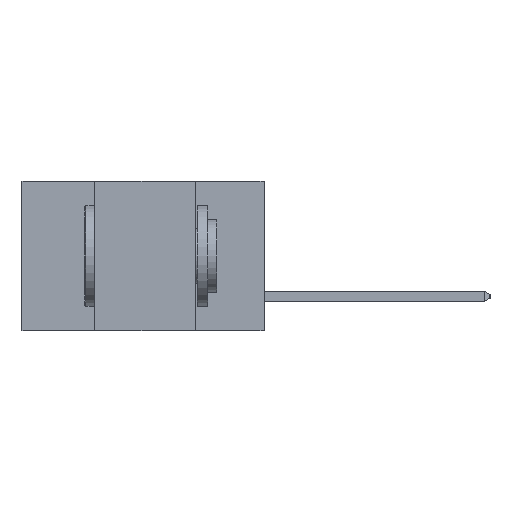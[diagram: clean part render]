
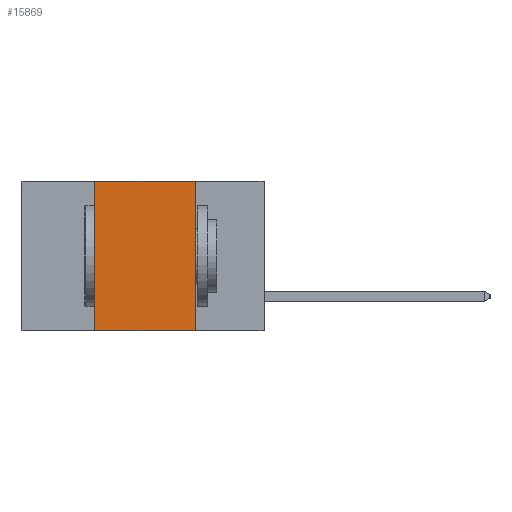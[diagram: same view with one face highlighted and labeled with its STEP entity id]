
A CAD part, left-side view. The second image highlights one B-rep face of the part: STEP entity #15869.
In plain terms, the highlighted planar face has unit normal (-1, 0, 0).
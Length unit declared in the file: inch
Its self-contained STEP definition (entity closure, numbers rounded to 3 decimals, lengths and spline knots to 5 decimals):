
#1483 = CARTESIAN_POINT ( 'NONE',  ( 0., 0.42, -0.37 ) ) ;
#1593 = DIRECTION ( 'NONE',  ( 0., 0., -1. ) ) ;
#1916 = LINE ( 'NONE', #15865, #14154 ) ;
#2330 = CARTESIAN_POINT ( 'NONE',  ( 0., 0.42, -0.37 ) ) ;
#3670 = VECTOR ( 'NONE', #6391, 39.37008 ) ;
#3976 = DIRECTION ( 'NONE',  ( 0., 0., 1. ) ) ;
#4157 = VECTOR ( 'NONE', #19181, 39.37008 ) ;
#5617 = CARTESIAN_POINT ( 'NONE',  ( 0., 0.17, 0. ) ) ;
#6391 = DIRECTION ( 'NONE',  ( 0., -1., 0. ) ) ;
#6900 = CARTESIAN_POINT ( 'NONE',  ( 0., 0.6, 0. ) ) ;
#7089 = ORIENTED_EDGE ( 'NONE', *, *, #11107, .F. ) ;
#7758 = VERTEX_POINT ( 'NONE', #15016 ) ;
#8998 = EDGE_CURVE ( 'NONE', #12867, #7758, #1916, .T. ) ;
#9630 = CARTESIAN_POINT ( 'NONE',  ( 0., 0.6, 0. ) ) ;
#10719 = VECTOR ( 'NONE', #3976, 39.37008 ) ;
#10819 = ORIENTED_EDGE ( 'NONE', *, *, #13196, .T. ) ;
#11107 = EDGE_CURVE ( 'NONE', #15363, #12867, #16710, .T. ) ;
#11159 = EDGE_LOOP ( 'NONE', ( #11821, #7089, #18902, #10819 ) ) ;
#11246 = DIRECTION ( 'NONE',  ( 1., 0., 0. ) ) ;
#11287 = DIRECTION ( 'NONE',  ( 0., 0., -1. ) ) ;
#11821 = ORIENTED_EDGE ( 'NONE', *, *, #8998, .F. ) ;
#12175 = EDGE_CURVE ( 'NONE', #18479, #15363, #15315, .T. ) ;
#12867 = VERTEX_POINT ( 'NONE', #5617 ) ;
#13196 = EDGE_CURVE ( 'NONE', #18479, #7758, #19892, .T. ) ;
#14154 = VECTOR ( 'NONE', #11287, 39.37008 ) ;
#15016 = CARTESIAN_POINT ( 'NONE',  ( 0., 0.17, -0.37 ) ) ;
#15315 = LINE ( 'NONE', #2330, #10719 ) ;
#15363 = VERTEX_POINT ( 'NONE', #17616 ) ;
#15865 = CARTESIAN_POINT ( 'NONE',  ( 0., 0.17, -0.37 ) ) ;
#15869 = ADVANCED_FACE ( 'NONE', ( #19815 ), #18808, .F. ) ;
#16710 = LINE ( 'NONE', #6900, #4157 ) ;
#17036 = AXIS2_PLACEMENT_3D ( 'NONE', #9630, #11246, #1593 ) ;
#17616 = CARTESIAN_POINT ( 'NONE',  ( 0., 0.42, 0. ) ) ;
#18479 = VERTEX_POINT ( 'NONE', #1483 ) ;
#18775 = CARTESIAN_POINT ( 'NONE',  ( 0., 0.6, -0.37 ) ) ;
#18808 = PLANE ( 'NONE',  #17036 ) ;
#18902 = ORIENTED_EDGE ( 'NONE', *, *, #12175, .F. ) ;
#19181 = DIRECTION ( 'NONE',  ( 0., -1., 0. ) ) ;
#19815 = FACE_OUTER_BOUND ( 'NONE', #11159, .T. ) ;
#19892 = LINE ( 'NONE', #18775, #3670 ) ;
